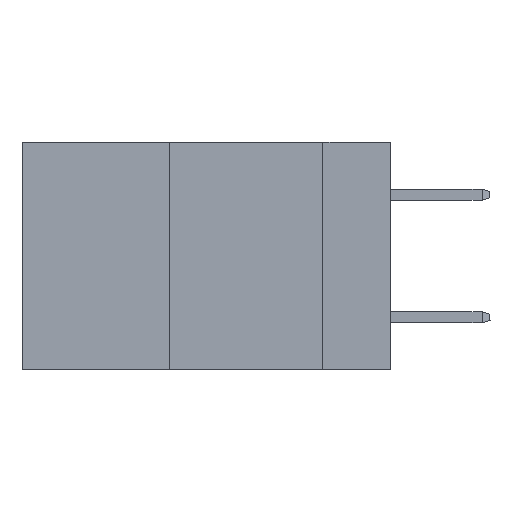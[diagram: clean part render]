
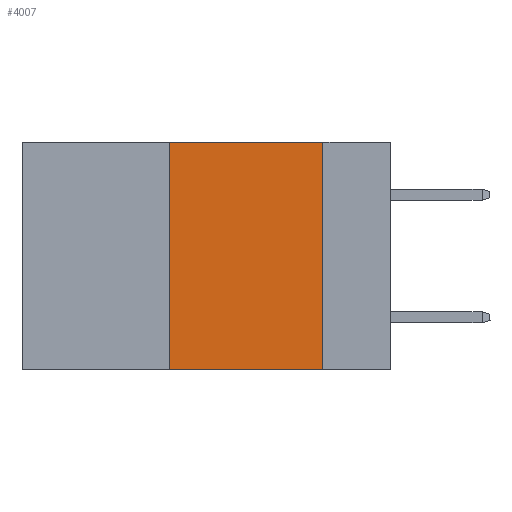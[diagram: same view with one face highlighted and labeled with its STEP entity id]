
A CAD part, left-side view. The second image highlights one B-rep face of the part: STEP entity #4007.
In plain terms, the highlighted planar face has unit normal (-1, 0, 0).
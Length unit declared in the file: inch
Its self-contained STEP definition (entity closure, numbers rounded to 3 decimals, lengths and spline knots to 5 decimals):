
#2137 = EDGE_CURVE ( 'NONE', #22276, #15671, #6221, .T. ) ;
#2618 = ORIENTED_EDGE ( 'NONE', *, *, #6527, .T. ) ;
#2702 = EDGE_LOOP ( 'NONE', ( #2809, #15958, #5225, #2618 ) ) ;
#2767 = DIRECTION ( 'NONE',  ( 1., 0., 0. ) ) ;
#2809 = ORIENTED_EDGE ( 'NONE', *, *, #2137, .F. ) ;
#3668 = DIRECTION ( 'NONE',  ( 0., -1., 0. ) ) ;
#3749 = CARTESIAN_POINT ( 'NONE',  ( 0., 0.36, -0.37 ) ) ;
#4007 = ADVANCED_FACE ( 'NONE', ( #13676 ), #23465, .F. ) ;
#5225 = ORIENTED_EDGE ( 'NONE', *, *, #15422, .F. ) ;
#5235 = DIRECTION ( 'NONE',  ( 0., -1., 0. ) ) ;
#5864 = CARTESIAN_POINT ( 'NONE',  ( 0., 0.11, -0.37 ) ) ;
#6221 = LINE ( 'NONE', #7950, #6241 ) ;
#6236 = CARTESIAN_POINT ( 'NONE',  ( 0., 0.6, 0. ) ) ;
#6241 = VECTOR ( 'NONE', #13785, 39.37008 ) ;
#6527 = EDGE_CURVE ( 'NONE', #20390, #15671, #18910, .T. ) ;
#6757 = CARTESIAN_POINT ( 'NONE',  ( 0., 0.36, 0. ) ) ;
#7950 = CARTESIAN_POINT ( 'NONE',  ( 0., 0.11, 0. ) ) ;
#7951 = VERTEX_POINT ( 'NONE', #6757 ) ;
#8049 = VECTOR ( 'NONE', #5235, 39.37008 ) ;
#8552 = CARTESIAN_POINT ( 'NONE',  ( 0., 0.11, 0. ) ) ;
#8617 = LINE ( 'NONE', #23620, #23723 ) ;
#13676 = FACE_OUTER_BOUND ( 'NONE', #2702, .T. ) ;
#13785 = DIRECTION ( 'NONE',  ( 0., 0., -1. ) ) ;
#14649 = LINE ( 'NONE', #22207, #8049 ) ;
#15422 = EDGE_CURVE ( 'NONE', #20390, #7951, #8617, .T. ) ;
#15671 = VERTEX_POINT ( 'NONE', #5864 ) ;
#15958 = ORIENTED_EDGE ( 'NONE', *, *, #22054, .F. ) ;
#17974 = VECTOR ( 'NONE', #3668, 39.37008 ) ;
#18910 = LINE ( 'NONE', #20293, #17974 ) ;
#19416 = AXIS2_PLACEMENT_3D ( 'NONE', #6236, #2767, #21358 ) ;
#20293 = CARTESIAN_POINT ( 'NONE',  ( 0., 0.6, -0.37 ) ) ;
#20390 = VERTEX_POINT ( 'NONE', #3749 ) ;
#21358 = DIRECTION ( 'NONE',  ( 0., 0., -1. ) ) ;
#21758 = DIRECTION ( 'NONE',  ( 0., 0., 1. ) ) ;
#22054 = EDGE_CURVE ( 'NONE', #7951, #22276, #14649, .T. ) ;
#22207 = CARTESIAN_POINT ( 'NONE',  ( 0., 0.6, 0. ) ) ;
#22276 = VERTEX_POINT ( 'NONE', #8552 ) ;
#23465 = PLANE ( 'NONE',  #19416 ) ;
#23620 = CARTESIAN_POINT ( 'NONE',  ( 0., 0.36, 0. ) ) ;
#23723 = VECTOR ( 'NONE', #21758, 39.37008 ) ;
